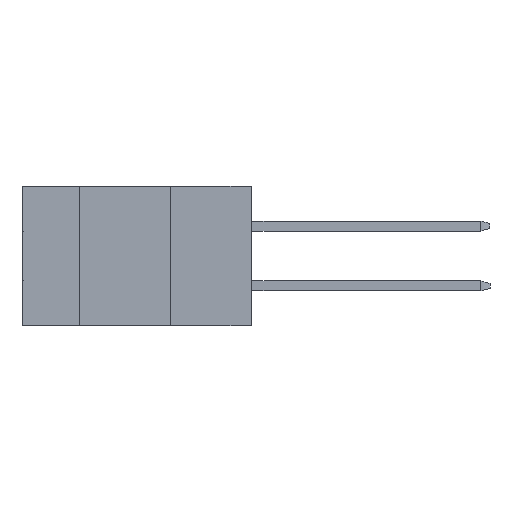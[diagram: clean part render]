
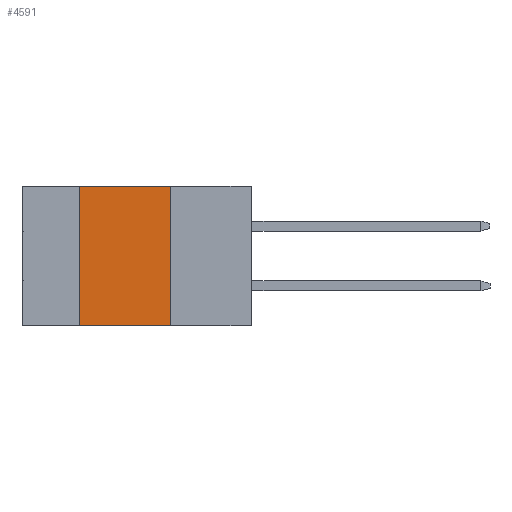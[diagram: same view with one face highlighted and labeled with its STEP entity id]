
A CAD part, left-side view. The second image highlights one B-rep face of the part: STEP entity #4591.
In plain terms, the highlighted planar face has unit normal (-1, 0, 0).
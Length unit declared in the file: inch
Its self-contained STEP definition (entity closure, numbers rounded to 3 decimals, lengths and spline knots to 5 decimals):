
#1423 = VERTEX_POINT ( 'NONE', #22363 ) ;
#2143 = DIRECTION ( 'NONE',  ( 0., 0., 1. ) ) ;
#3154 = VECTOR ( 'NONE', #2143, 39.37008 ) ;
#3575 = LINE ( 'NONE', #12668, #14322 ) ;
#4591 = ADVANCED_FACE ( 'NONE', ( #14446 ), #21851, .F. ) ;
#5217 = CARTESIAN_POINT ( 'NONE',  ( 0., 0.254, 0. ) ) ;
#5466 = EDGE_CURVE ( 'NONE', #1423, #16014, #7597, .T. ) ;
#6239 = VERTEX_POINT ( 'NONE', #6926 ) ;
#6926 = CARTESIAN_POINT ( 'NONE',  ( 0., 0.254, -0.437 ) ) ;
#7322 = EDGE_CURVE ( 'NONE', #1423, #6239, #20648, .T. ) ;
#7597 = LINE ( 'NONE', #15013, #3154 ) ;
#8779 = DIRECTION ( 'NONE',  ( 0., 0., -1. ) ) ;
#9422 = ORIENTED_EDGE ( 'NONE', *, *, #5466, .F. ) ;
#10670 = CARTESIAN_POINT ( 'NONE',  ( 0., 0.72, 0. ) ) ;
#10972 = VECTOR ( 'NONE', #19354, 39.37008 ) ;
#12087 = EDGE_LOOP ( 'NONE', ( #22234, #19915, #9422, #18012 ) ) ;
#12668 = CARTESIAN_POINT ( 'NONE',  ( 0., 0.254, -0.437 ) ) ;
#14322 = VECTOR ( 'NONE', #8779, 39.37008 ) ;
#14446 = FACE_OUTER_BOUND ( 'NONE', #12087, .T. ) ;
#14819 = DIRECTION ( 'NONE',  ( 0., 0., -1. ) ) ;
#14823 = EDGE_CURVE ( 'NONE', #20678, #6239, #3575, .T. ) ;
#15013 = CARTESIAN_POINT ( 'NONE',  ( 0., 0.54, -0.437 ) ) ;
#15441 = DIRECTION ( 'NONE',  ( 0., -1., 0. ) ) ;
#16014 = VERTEX_POINT ( 'NONE', #20854 ) ;
#17145 = AXIS2_PLACEMENT_3D ( 'NONE', #10670, #23882, #14819 ) ;
#17540 = LINE ( 'NONE', #17774, #10972 ) ;
#17774 = CARTESIAN_POINT ( 'NONE',  ( 0., 0.72, 0. ) ) ;
#18012 = ORIENTED_EDGE ( 'NONE', *, *, #7322, .T. ) ;
#18953 = CARTESIAN_POINT ( 'NONE',  ( 0., 0.72, -0.437 ) ) ;
#19354 = DIRECTION ( 'NONE',  ( 0., -1., 0. ) ) ;
#19915 = ORIENTED_EDGE ( 'NONE', *, *, #21450, .F. ) ;
#20648 = LINE ( 'NONE', #18953, #23736 ) ;
#20678 = VERTEX_POINT ( 'NONE', #5217 ) ;
#20854 = CARTESIAN_POINT ( 'NONE',  ( 0., 0.54, 0. ) ) ;
#21450 = EDGE_CURVE ( 'NONE', #16014, #20678, #17540, .T. ) ;
#21851 = PLANE ( 'NONE',  #17145 ) ;
#22234 = ORIENTED_EDGE ( 'NONE', *, *, #14823, .F. ) ;
#22363 = CARTESIAN_POINT ( 'NONE',  ( 0., 0.54, -0.437 ) ) ;
#23736 = VECTOR ( 'NONE', #15441, 39.37008 ) ;
#23882 = DIRECTION ( 'NONE',  ( 1., 0., 0. ) ) ;
